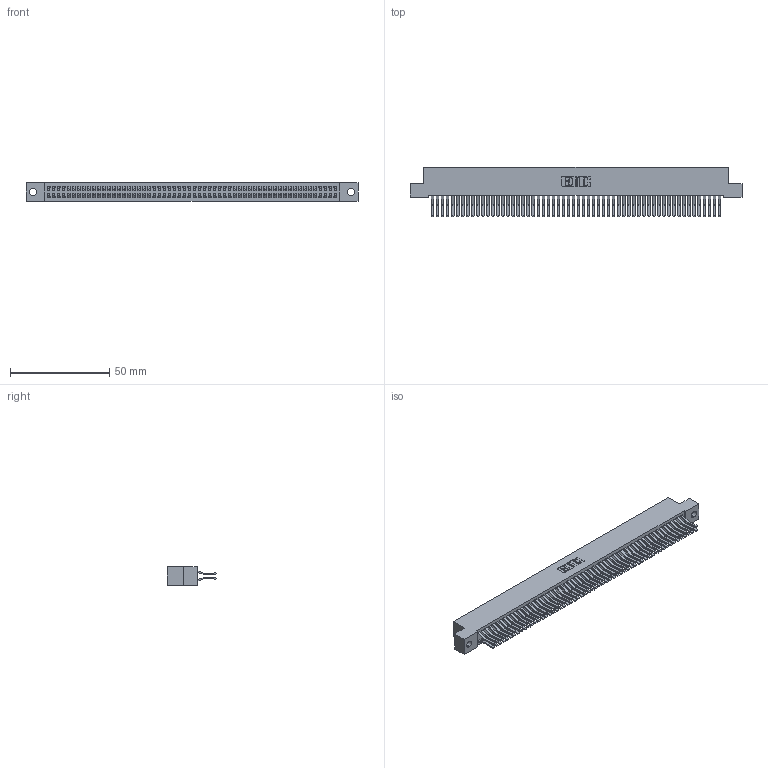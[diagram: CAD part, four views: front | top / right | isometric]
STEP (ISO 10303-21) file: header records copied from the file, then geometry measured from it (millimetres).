
FILE_DESCRIPTION (( 'STEP AP203' ), '1' );
FILE_NAME ('392-116-560-202.STEP', '2019-10-10T02:06:44', ( '' ), ( '' ), 'SwSTEP 2.0', 'SolidWorks 2016', '' );
FILE_SCHEMA (( 'CONFIG_CONTROL_DESIGN' ));
Length unit declared in the file: inch
Products named in the file (3): 342 Part_.128 Slot; 345-292-001_560 Tail; 392-116-560-202
Assembly tree (117 placements, depth 2):
  392-116-560-202
    342 Part_.128 Slot
    345-292-001_560 Tail  x116
Bounding box: 167.64 x 24.78 x 9.4 mm (x, y, z)
Volume: 15847.6 mm3; surface area: 27775.8 mm2
Topology: 117 solids, 117 shells, 6378 faces, 18987 edges, 12502 vertices
Faces by surface type: plane 4246, cylinder 2132
Entity records: 35335 total; most frequent: CARTESIAN_POINT 5838, ORIENTED_EDGE 5774, DIRECTION 4963, EDGE_CURVE 2887, LINE 2755, VECTOR 2755, VERTEX_POINT 1922, AXIS2_PLACEMENT_3D 1104
